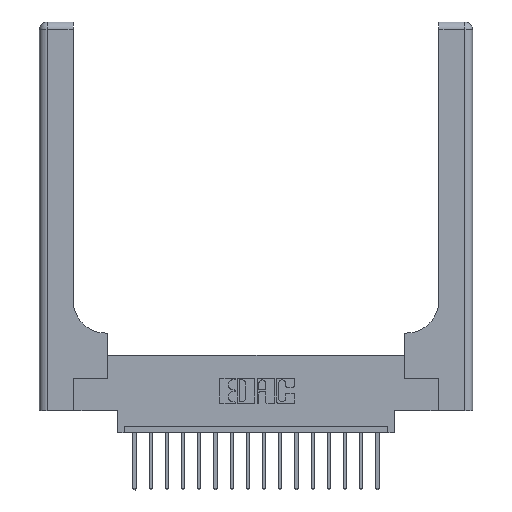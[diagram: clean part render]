
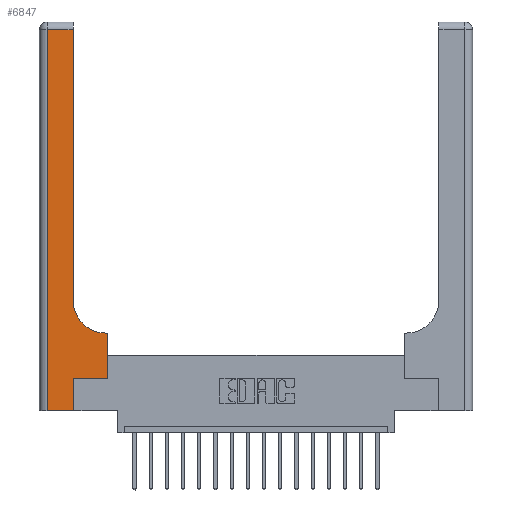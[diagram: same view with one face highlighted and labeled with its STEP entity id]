
A CAD part, top view. The second image highlights one B-rep face of the part: STEP entity #6847.
In plain terms, the highlighted planar face has unit normal (0, 0, 1).
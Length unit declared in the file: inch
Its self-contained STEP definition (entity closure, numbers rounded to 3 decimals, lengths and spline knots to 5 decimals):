
#160 = VERTEX_POINT ( 'NONE', #10359 ) ;
#558 = LINE ( 'NONE', #8110, #16917 ) ;
#1106 = DIRECTION ( 'NONE',  ( -1., 0., 0. ) ) ;
#1143 = VERTEX_POINT ( 'NONE', #3861 ) ;
#1303 = CARTESIAN_POINT ( 'NONE',  ( 0.51, 0.85, 0.37 ) ) ;
#1377 = CARTESIAN_POINT ( 'NONE',  ( 0.265, 0., 0.37 ) ) ;
#1464 = DIRECTION ( 'NONE',  ( 0., -1., 0. ) ) ;
#1543 = EDGE_LOOP ( 'NONE', ( #11044, #14671, #17165, #5084, #6657, #11604, #10601, #3318, #9559 ) ) ;
#1771 = LINE ( 'NONE', #17860, #8410 ) ;
#1905 = VERTEX_POINT ( 'NONE', #18700 ) ;
#2026 = VERTEX_POINT ( 'NONE', #17797 ) ;
#2148 = VECTOR ( 'NONE', #16717, 39.37008 ) ;
#2403 = CARTESIAN_POINT ( 'NONE',  ( 0.26, 2.94, 0.37 ) ) ;
#2564 = CARTESIAN_POINT ( 'NONE',  ( 0., 2.94, 0.37 ) ) ;
#3256 = CARTESIAN_POINT ( 'NONE',  ( 0.528, 0.25, 0.37 ) ) ;
#3318 = ORIENTED_EDGE ( 'NONE', *, *, #12566, .T. ) ;
#3326 = PLANE ( 'NONE',  #6429 ) ;
#3861 = CARTESIAN_POINT ( 'NONE',  ( 0.06, 2.94, 0.37 ) ) ;
#4832 = DIRECTION ( 'NONE',  ( -1., 0., 0. ) ) ;
#5084 = ORIENTED_EDGE ( 'NONE', *, *, #7741, .T. ) ;
#5142 = FACE_OUTER_BOUND ( 'NONE', #1543, .T. ) ;
#5689 = CARTESIAN_POINT ( 'NONE',  ( 0.265, 0., 0.37 ) ) ;
#6041 = VERTEX_POINT ( 'NONE', #14830 ) ;
#6429 = AXIS2_PLACEMENT_3D ( 'NONE', #13521, #17654, #4832 ) ;
#6657 = ORIENTED_EDGE ( 'NONE', *, *, #17659, .T. ) ;
#6847 = ADVANCED_FACE ( 'NONE', ( #5142 ), #3326, .F. ) ;
#7130 = EDGE_CURVE ( 'NONE', #160, #1905, #558, .T. ) ;
#7741 = EDGE_CURVE ( 'NONE', #15467, #12829, #17118, .T. ) ;
#8034 = CIRCLE ( 'NONE', #12164, 0.25 ) ;
#8110 = CARTESIAN_POINT ( 'NONE',  ( 0.265, 0.25, 0.37 ) ) ;
#8182 = CARTESIAN_POINT ( 'NONE',  ( 0., 0., 0.37 ) ) ;
#8410 = VECTOR ( 'NONE', #14784, 39.37008 ) ;
#9021 = LINE ( 'NONE', #1377, #16265 ) ;
#9067 = CARTESIAN_POINT ( 'NONE',  ( 0.528, 0.6, 0.37 ) ) ;
#9408 = EDGE_CURVE ( 'NONE', #6041, #12115, #1771, .T. ) ;
#9559 = ORIENTED_EDGE ( 'NONE', *, *, #13966, .T. ) ;
#10188 = DIRECTION ( 'NONE',  ( 1., 0., 0. ) ) ;
#10359 = CARTESIAN_POINT ( 'NONE',  ( 0.265, 0.25, 0.37 ) ) ;
#10601 = ORIENTED_EDGE ( 'NONE', *, *, #16059, .T. ) ;
#10603 = VECTOR ( 'NONE', #1464, 39.37008 ) ;
#10768 = DIRECTION ( 'NONE',  ( 0., 1., 0. ) ) ;
#10799 = LINE ( 'NONE', #18094, #2148 ) ;
#11044 = ORIENTED_EDGE ( 'NONE', *, *, #9408, .T. ) ;
#11224 = DIRECTION ( 'NONE',  ( 1., 0., 0. ) ) ;
#11604 = ORIENTED_EDGE ( 'NONE', *, *, #7130, .T. ) ;
#12115 = VERTEX_POINT ( 'NONE', #2403 ) ;
#12164 = AXIS2_PLACEMENT_3D ( 'NONE', #1303, #12961, #10188 ) ;
#12566 = EDGE_CURVE ( 'NONE', #16116, #2026, #10799, .T. ) ;
#12829 = VERTEX_POINT ( 'NONE', #5689 ) ;
#12961 = DIRECTION ( 'NONE',  ( 0., 0., -1. ) ) ;
#13521 = CARTESIAN_POINT ( 'NONE',  ( 0., 3., 0.37 ) ) ;
#13574 = LINE ( 'NONE', #18791, #10603 ) ;
#13966 = EDGE_CURVE ( 'NONE', #2026, #6041, #8034, .T. ) ;
#14453 = DIRECTION ( 'NONE',  ( 0., 1., 0. ) ) ;
#14671 = ORIENTED_EDGE ( 'NONE', *, *, #18307, .T. ) ;
#14784 = DIRECTION ( 'NONE',  ( 0., 1., 0. ) ) ;
#14830 = CARTESIAN_POINT ( 'NONE',  ( 0.26, 0.85, 0.37 ) ) ;
#14863 = VECTOR ( 'NONE', #1106, 39.37008 ) ;
#15218 = CARTESIAN_POINT ( 'NONE',  ( 0.06, 0., 0.37 ) ) ;
#15467 = VERTEX_POINT ( 'NONE', #15218 ) ;
#16006 = LINE ( 'NONE', #2564, #14863 ) ;
#16059 = EDGE_CURVE ( 'NONE', #1905, #16116, #17196, .T. ) ;
#16116 = VERTEX_POINT ( 'NONE', #9067 ) ;
#16265 = VECTOR ( 'NONE', #14453, 39.37008 ) ;
#16519 = VECTOR ( 'NONE', #10768, 39.37008 ) ;
#16717 = DIRECTION ( 'NONE',  ( -1., 0., 0. ) ) ;
#16917 = VECTOR ( 'NONE', #18070, 39.37008 ) ;
#17118 = LINE ( 'NONE', #8182, #18465 ) ;
#17165 = ORIENTED_EDGE ( 'NONE', *, *, #17218, .T. ) ;
#17196 = LINE ( 'NONE', #3256, #16519 ) ;
#17218 = EDGE_CURVE ( 'NONE', #1143, #15467, #13574, .T. ) ;
#17654 = DIRECTION ( 'NONE',  ( 0., 0., -1. ) ) ;
#17659 = EDGE_CURVE ( 'NONE', #12829, #160, #9021, .T. ) ;
#17797 = CARTESIAN_POINT ( 'NONE',  ( 0.51, 0.6, 0.37 ) ) ;
#17860 = CARTESIAN_POINT ( 'NONE',  ( 0.26, 3., 0.37 ) ) ;
#18070 = DIRECTION ( 'NONE',  ( 1., 0., 0. ) ) ;
#18094 = CARTESIAN_POINT ( 'NONE',  ( 0.26, 0.6, 0.37 ) ) ;
#18307 = EDGE_CURVE ( 'NONE', #12115, #1143, #16006, .T. ) ;
#18465 = VECTOR ( 'NONE', #11224, 39.37008 ) ;
#18700 = CARTESIAN_POINT ( 'NONE',  ( 0.528, 0.25, 0.37 ) ) ;
#18791 = CARTESIAN_POINT ( 'NONE',  ( 0.06, 3., 0.37 ) ) ;
